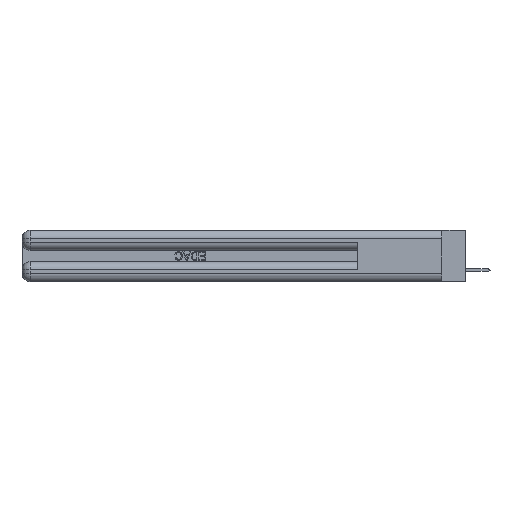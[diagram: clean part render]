
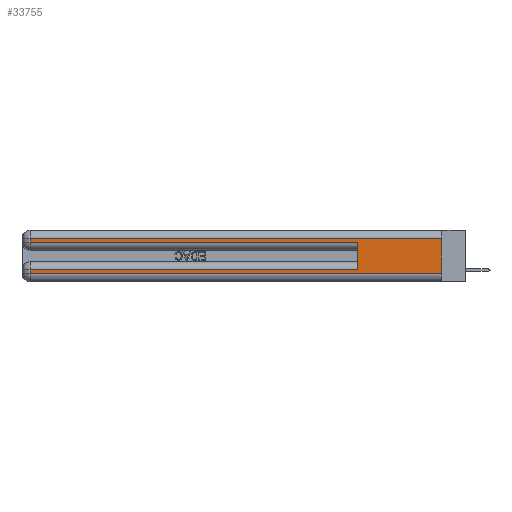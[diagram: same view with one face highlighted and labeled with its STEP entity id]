
A CAD part, left-side view. The second image highlights one B-rep face of the part: STEP entity #33755.
In plain terms, the highlighted planar face has unit normal (-1, 0, 0).
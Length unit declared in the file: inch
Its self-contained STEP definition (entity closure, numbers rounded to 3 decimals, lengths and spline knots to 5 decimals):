
#235 = CARTESIAN_POINT ( 'NONE',  ( 0., 0., 0.37 ) ) ;
#341 = CARTESIAN_POINT ( 'NONE',  ( 0., 2.94, 0.285 ) ) ;
#2284 = ORIENTED_EDGE ( 'NONE', *, *, #11925, .T. ) ;
#2455 = DIRECTION ( 'NONE',  ( 0., 1., 0. ) ) ;
#2562 = LINE ( 'NONE', #22987, #39646 ) ;
#2704 = CARTESIAN_POINT ( 'NONE',  ( 0., 0., 0.06 ) ) ;
#2720 = EDGE_CURVE ( 'NONE', #36756, #46179, #13942, .T. ) ;
#5332 = DIRECTION ( 'NONE',  ( 0., 1., 0. ) ) ;
#5608 = ORIENTED_EDGE ( 'NONE', *, *, #10111, .T. ) ;
#6161 = VECTOR ( 'NONE', #14203, 39.37008 ) ;
#6685 = EDGE_CURVE ( 'NONE', #49849, #22013, #6849, .T. ) ;
#6810 = ORIENTED_EDGE ( 'NONE', *, *, #31985, .T. ) ;
#6849 = LINE ( 'NONE', #29191, #16676 ) ;
#7378 = CARTESIAN_POINT ( 'NONE',  ( 0., 0., 0.285 ) ) ;
#7453 = VECTOR ( 'NONE', #27320, 39.37008 ) ;
#8722 = VECTOR ( 'NONE', #19434, 39.37008 ) ;
#9457 = VERTEX_POINT ( 'NONE', #12333 ) ;
#9807 = ORIENTED_EDGE ( 'NONE', *, *, #6685, .F. ) ;
#10111 = EDGE_CURVE ( 'NONE', #49849, #34921, #17507, .T. ) ;
#11826 = DIRECTION ( 'NONE',  ( 0., 0., -1. ) ) ;
#11925 = EDGE_CURVE ( 'NONE', #25767, #22013, #28420, .T. ) ;
#12333 = CARTESIAN_POINT ( 'NONE',  ( 0., 0., 0.31 ) ) ;
#12918 = LINE ( 'NONE', #13168, #6161 ) ;
#13168 = CARTESIAN_POINT ( 'NONE',  ( 0., 0., 0.37 ) ) ;
#13942 = LINE ( 'NONE', #2704, #29941 ) ;
#14203 = DIRECTION ( 'NONE',  ( 0., 0., -1. ) ) ;
#15225 = DIRECTION ( 'NONE',  ( 0., 0., -1. ) ) ;
#15735 = CARTESIAN_POINT ( 'NONE',  ( 0., 0., 0.06 ) ) ;
#16398 = CARTESIAN_POINT ( 'NONE',  ( 0., 2.94, 0.06 ) ) ;
#16676 = VECTOR ( 'NONE', #33170, 39.37008 ) ;
#17507 = LINE ( 'NONE', #36916, #22483 ) ;
#18360 = EDGE_CURVE ( 'NONE', #9457, #46179, #12918, .T. ) ;
#19434 = DIRECTION ( 'NONE',  ( 0., -1., 0. ) ) ;
#19661 = CARTESIAN_POINT ( 'NONE',  ( 0., 2.94, 0.31 ) ) ;
#19875 = CARTESIAN_POINT ( 'NONE',  ( 0., 2.94, 0.37 ) ) ;
#21909 = ORIENTED_EDGE ( 'NONE', *, *, #32339, .T. ) ;
#22013 = VERTEX_POINT ( 'NONE', #26501 ) ;
#22483 = VECTOR ( 'NONE', #5332, 39.37008 ) ;
#22987 = CARTESIAN_POINT ( 'NONE',  ( 0., 2.94, 0.37 ) ) ;
#25767 = VERTEX_POINT ( 'NONE', #341 ) ;
#26501 = CARTESIAN_POINT ( 'NONE',  ( 0., 0.6, 0.285 ) ) ;
#27320 = DIRECTION ( 'NONE',  ( 0., 0., -1. ) ) ;
#28420 = LINE ( 'NONE', #7378, #8722 ) ;
#29191 = CARTESIAN_POINT ( 'NONE',  ( 0., 0.6, 0.145 ) ) ;
#29941 = VECTOR ( 'NONE', #49336, 39.37008 ) ;
#31819 = ORIENTED_EDGE ( 'NONE', *, *, #2720, .T. ) ;
#31985 = EDGE_CURVE ( 'NONE', #34921, #36756, #2562, .T. ) ;
#32339 = EDGE_CURVE ( 'NONE', #9457, #34418, #45801, .T. ) ;
#33170 = DIRECTION ( 'NONE',  ( 0., 0., 1. ) ) ;
#33755 = ADVANCED_FACE ( 'NONE', ( #39430 ), #35470, .F. ) ;
#34418 = VERTEX_POINT ( 'NONE', #19661 ) ;
#34833 = CARTESIAN_POINT ( 'NONE',  ( 0., 0.6, 0.085 ) ) ;
#34921 = VERTEX_POINT ( 'NONE', #50777 ) ;
#35470 = PLANE ( 'NONE',  #45914 ) ;
#35649 = EDGE_CURVE ( 'NONE', #34418, #25767, #47033, .T. ) ;
#35804 = DIRECTION ( 'NONE',  ( 1., 0., 0. ) ) ;
#36601 = CARTESIAN_POINT ( 'NONE',  ( 0., 0., 0.31 ) ) ;
#36756 = VERTEX_POINT ( 'NONE', #16398 ) ;
#36916 = CARTESIAN_POINT ( 'NONE',  ( 0., 0., 0.085 ) ) ;
#39430 = FACE_OUTER_BOUND ( 'NONE', #47327, .T. ) ;
#39646 = VECTOR ( 'NONE', #15225, 39.37008 ) ;
#40808 = VECTOR ( 'NONE', #2455, 39.37008 ) ;
#44867 = ORIENTED_EDGE ( 'NONE', *, *, #35649, .T. ) ;
#45801 = LINE ( 'NONE', #36601, #40808 ) ;
#45914 = AXIS2_PLACEMENT_3D ( 'NONE', #235, #35804, #11826 ) ;
#46179 = VERTEX_POINT ( 'NONE', #15735 ) ;
#47033 = LINE ( 'NONE', #19875, #7453 ) ;
#47327 = EDGE_LOOP ( 'NONE', ( #50156, #21909, #44867, #2284, #9807, #5608, #6810, #31819 ) ) ;
#49336 = DIRECTION ( 'NONE',  ( 0., -1., 0. ) ) ;
#49849 = VERTEX_POINT ( 'NONE', #34833 ) ;
#50156 = ORIENTED_EDGE ( 'NONE', *, *, #18360, .F. ) ;
#50777 = CARTESIAN_POINT ( 'NONE',  ( 0., 2.94, 0.085 ) ) ;
